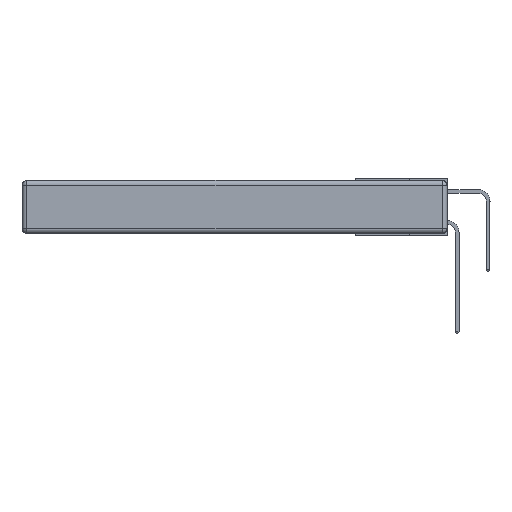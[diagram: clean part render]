
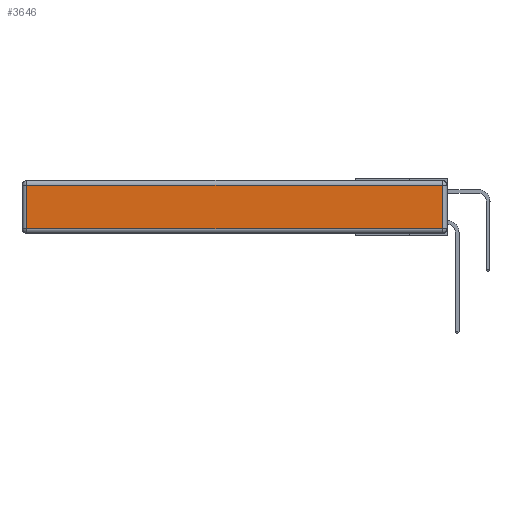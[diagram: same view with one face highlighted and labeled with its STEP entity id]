
A CAD part, left-side view. The second image highlights one B-rep face of the part: STEP entity #3646.
In plain terms, the highlighted planar face has unit normal (-1, 0, 0).
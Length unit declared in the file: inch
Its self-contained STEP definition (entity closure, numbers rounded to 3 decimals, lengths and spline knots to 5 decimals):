
#411 = FACE_OUTER_BOUND ( 'NONE', #12793, .T. ) ;
#1594 = CARTESIAN_POINT ( 'NONE',  ( 0., 2.72, -0.343 ) ) ;
#1853 = CARTESIAN_POINT ( 'NONE',  ( 0., 0.03, -0.343 ) ) ;
#1966 = EDGE_CURVE ( 'NONE', #26016, #33609, #36278, .T. ) ;
#2949 = ORIENTED_EDGE ( 'NONE', *, *, #35663, .T. ) ;
#3331 = VERTEX_POINT ( 'NONE', #32415 ) ;
#3347 = VECTOR ( 'NONE', #35830, 39.37008 ) ;
#3646 = ADVANCED_FACE ( 'NONE', ( #411 ), #10557, .T. ) ;
#3816 = DIRECTION ( 'NONE',  ( 0., 0., 1. ) ) ;
#6057 = ORIENTED_EDGE ( 'NONE', *, *, #15280, .T. ) ;
#7265 = DIRECTION ( 'NONE',  ( 0., -1., 0. ) ) ;
#7741 = ORIENTED_EDGE ( 'NONE', *, *, #1966, .T. ) ;
#10557 = PLANE ( 'NONE',  #27555 ) ;
#10910 = DIRECTION ( 'NONE',  ( 0., 0., 1. ) ) ;
#11251 = CARTESIAN_POINT ( 'NONE',  ( 0., 2.75, -0.03 ) ) ;
#11431 = EDGE_CURVE ( 'NONE', #33609, #3331, #20843, .T. ) ;
#12189 = LINE ( 'NONE', #1594, #3347 ) ;
#12793 = EDGE_LOOP ( 'NONE', ( #2949, #7741, #35450, #6057 ) ) ;
#15280 = EDGE_CURVE ( 'NONE', #3331, #32703, #12189, .T. ) ;
#17525 = CARTESIAN_POINT ( 'NONE',  ( 0., 2.72, -0.313 ) ) ;
#17631 = CARTESIAN_POINT ( 'NONE',  ( 0., 0.03, -0.313 ) ) ;
#19065 = VECTOR ( 'NONE', #33411, 39.37008 ) ;
#20843 = LINE ( 'NONE', #11251, #19065 ) ;
#21335 = VECTOR ( 'NONE', #3816, 39.37008 ) ;
#22002 = CARTESIAN_POINT ( 'NONE',  ( 0., 0., -0.343 ) ) ;
#22130 = DIRECTION ( 'NONE',  ( -1., 0., 0. ) ) ;
#23203 = VECTOR ( 'NONE', #7265, 39.37008 ) ;
#24146 = CARTESIAN_POINT ( 'NONE',  ( 0., 0., -0.313 ) ) ;
#24581 = CARTESIAN_POINT ( 'NONE',  ( 0., 0.03, -0.03 ) ) ;
#26016 = VERTEX_POINT ( 'NONE', #17631 ) ;
#27555 = AXIS2_PLACEMENT_3D ( 'NONE', #22002, #22130, #10910 ) ;
#32415 = CARTESIAN_POINT ( 'NONE',  ( 0., 2.72, -0.03 ) ) ;
#32703 = VERTEX_POINT ( 'NONE', #17525 ) ;
#32869 = LINE ( 'NONE', #24146, #23203 ) ;
#33411 = DIRECTION ( 'NONE',  ( 0., 1., 0. ) ) ;
#33609 = VERTEX_POINT ( 'NONE', #24581 ) ;
#35450 = ORIENTED_EDGE ( 'NONE', *, *, #11431, .T. ) ;
#35663 = EDGE_CURVE ( 'NONE', #32703, #26016, #32869, .T. ) ;
#35830 = DIRECTION ( 'NONE',  ( 0., 0., -1. ) ) ;
#36278 = LINE ( 'NONE', #1853, #21335 ) ;
